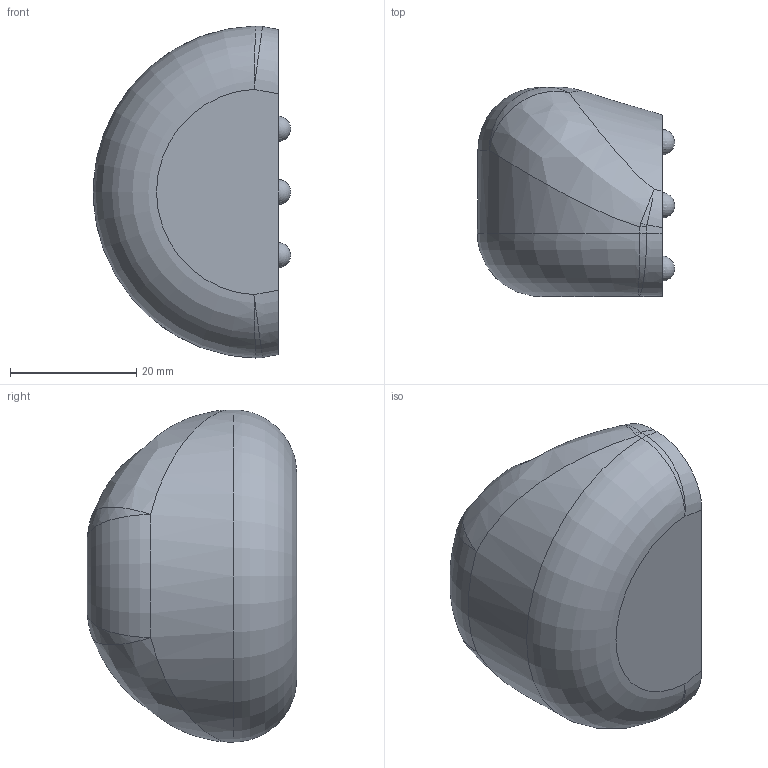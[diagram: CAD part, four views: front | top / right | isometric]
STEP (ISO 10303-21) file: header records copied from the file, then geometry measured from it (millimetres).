
FILE_DESCRIPTION (( 'STEP AP214' ), '1' );
FILE_NAME ('Stock_Knob_V2.step', '2016-01-25T18:17:26', ( 'WarFairy' ), ( '' ), 'SwSTEP 2.0', 'SolidWorks 2015', '' );
FILE_SCHEMA (( 'AUTOMOTIVE_DESIGN' ));
Length unit declared in the file: millimetre
Products named in the file (1): Stock_Knob_V2
Bounding box: 31.21 x 33.09 x 52.53 mm (x, y, z)
Volume: 32914 mm3; surface area: 5586 mm2
Topology: 1 solids, 1 shells, 30 faces, 74 edges, 38 vertices
Faces by surface type: bspline 11, sphere 6, torus 5, cylinder 5, plane 3
Entity records: 1492 total; most frequent: CARTESIAN_POINT 922, ORIENTED_EDGE 116, DIRECTION 97, EDGE_CURVE 58, AXIS2_PLACEMENT_3D 45, VERTEX_POINT 34, EDGE_LOOP 34, FACE_OUTER_BOUND 30
